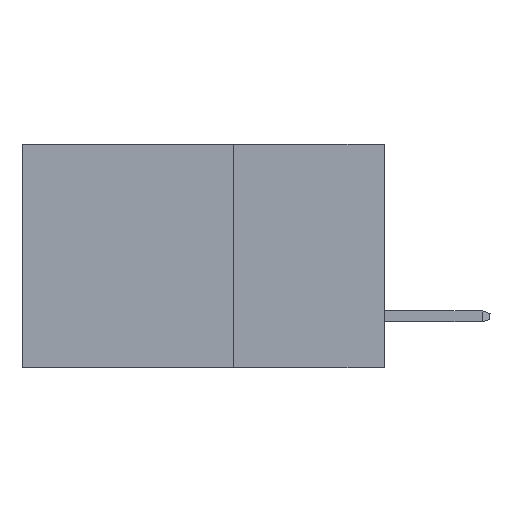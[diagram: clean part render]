
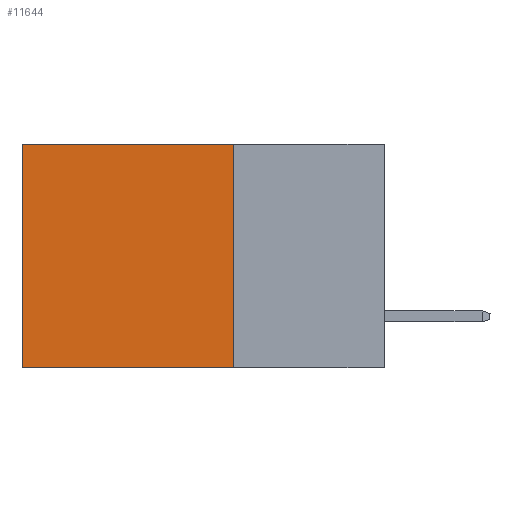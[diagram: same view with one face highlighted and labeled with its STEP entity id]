
A CAD part, left-side view. The second image highlights one B-rep face of the part: STEP entity #11644.
In plain terms, the highlighted planar face has unit normal (-1, 0, 0).
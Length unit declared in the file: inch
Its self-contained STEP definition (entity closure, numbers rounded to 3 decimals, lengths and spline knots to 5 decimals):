
#120 = EDGE_CURVE ( 'NONE', #20716, #5325, #1890, .T. ) ;
#283 = CARTESIAN_POINT ( 'NONE',  ( 0.298, 0.25, 0. ) ) ;
#506 = VECTOR ( 'NONE', #9313, 39.37008 ) ;
#1890 = LINE ( 'NONE', #22376, #16413 ) ;
#2209 = VERTEX_POINT ( 'NONE', #11986 ) ;
#3717 = DIRECTION ( 'NONE',  ( 0., 0., -1. ) ) ;
#4011 = DIRECTION ( 'NONE',  ( 0., 1., 0. ) ) ;
#4427 = DIRECTION ( 'NONE',  ( 1., 0., 0. ) ) ;
#5122 = CARTESIAN_POINT ( 'NONE',  ( 0.298, 0.25, -0.37 ) ) ;
#5215 = EDGE_LOOP ( 'NONE', ( #18263, #11224, #10747, #11466 ) ) ;
#5325 = VERTEX_POINT ( 'NONE', #11649 ) ;
#5518 = LINE ( 'NONE', #10911, #506 ) ;
#6114 = CARTESIAN_POINT ( 'NONE',  ( 0.298, 0.25, 0. ) ) ;
#6951 = VECTOR ( 'NONE', #23231, 39.37008 ) ;
#7620 = EDGE_CURVE ( 'NONE', #2209, #11928, #5518, .T. ) ;
#8098 = PLANE ( 'NONE',  #20328 ) ;
#9313 = DIRECTION ( 'NONE',  ( 0., 0., -1. ) ) ;
#10747 = ORIENTED_EDGE ( 'NONE', *, *, #7620, .F. ) ;
#10911 = CARTESIAN_POINT ( 'NONE',  ( 0.298, 0.25, 0. ) ) ;
#11093 = EDGE_CURVE ( 'NONE', #2209, #20716, #13699, .T. ) ;
#11224 = ORIENTED_EDGE ( 'NONE', *, *, #22260, .F. ) ;
#11466 = ORIENTED_EDGE ( 'NONE', *, *, #11093, .T. ) ;
#11638 = DIRECTION ( 'NONE',  ( 0., 0., -1. ) ) ;
#11644 = ADVANCED_FACE ( 'NONE', ( #20040 ), #8098, .F. ) ;
#11649 = CARTESIAN_POINT ( 'NONE',  ( 0.298, 0.6, -0.37 ) ) ;
#11928 = VERTEX_POINT ( 'NONE', #5122 ) ;
#11986 = CARTESIAN_POINT ( 'NONE',  ( 0.298, 0.25, 0. ) ) ;
#13699 = LINE ( 'NONE', #283, #14267 ) ;
#13714 = CARTESIAN_POINT ( 'NONE',  ( 0.298, 0.25, -0.37 ) ) ;
#14267 = VECTOR ( 'NONE', #4011, 39.37008 ) ;
#16413 = VECTOR ( 'NONE', #3717, 39.37008 ) ;
#18263 = ORIENTED_EDGE ( 'NONE', *, *, #120, .T. ) ;
#19101 = CARTESIAN_POINT ( 'NONE',  ( 0.298, 0.6, 0. ) ) ;
#20040 = FACE_OUTER_BOUND ( 'NONE', #5215, .T. ) ;
#20328 = AXIS2_PLACEMENT_3D ( 'NONE', #6114, #4427, #11638 ) ;
#20716 = VERTEX_POINT ( 'NONE', #19101 ) ;
#22260 = EDGE_CURVE ( 'NONE', #11928, #5325, #22702, .T. ) ;
#22376 = CARTESIAN_POINT ( 'NONE',  ( 0.298, 0.6, 0. ) ) ;
#22702 = LINE ( 'NONE', #13714, #6951 ) ;
#23231 = DIRECTION ( 'NONE',  ( 0., 1., 0. ) ) ;
